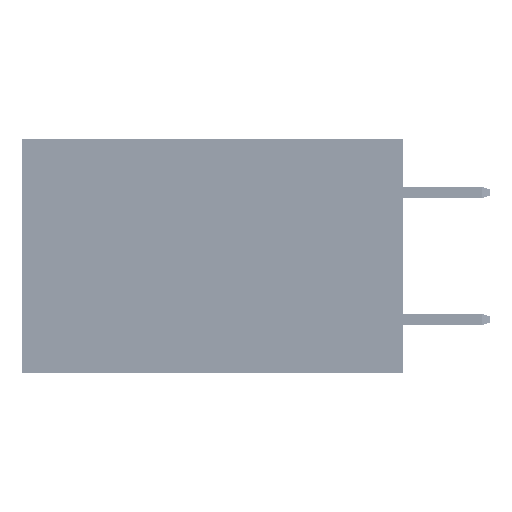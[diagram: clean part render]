
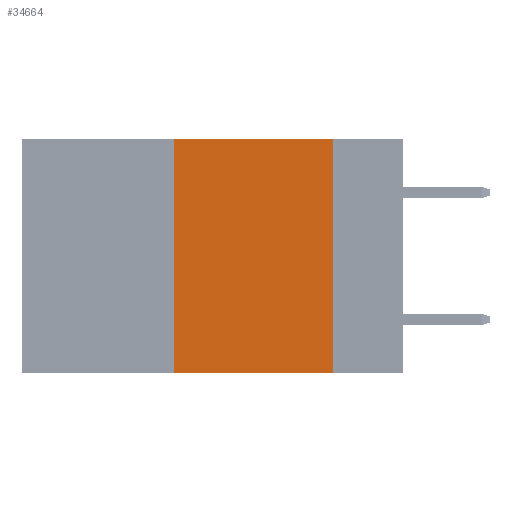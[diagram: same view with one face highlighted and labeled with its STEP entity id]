
A CAD part, left-side view. The second image highlights one B-rep face of the part: STEP entity #34664.
In plain terms, the highlighted planar face has unit normal (-1, 0, 0).
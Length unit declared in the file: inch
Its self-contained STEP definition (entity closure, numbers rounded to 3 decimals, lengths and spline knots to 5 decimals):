
#828 = CARTESIAN_POINT ( 'NONE',  ( 0., 0.11, -0.37 ) ) ;
#5156 = VERTEX_POINT ( 'NONE', #828 ) ;
#6216 = LINE ( 'NONE', #47493, #41495 ) ;
#6456 = DIRECTION ( 'NONE',  ( 0., 0., -1. ) ) ;
#7504 = DIRECTION ( 'NONE',  ( 0., -1., 0. ) ) ;
#7778 = DIRECTION ( 'NONE',  ( 0., 0., 1. ) ) ;
#10193 = DIRECTION ( 'NONE',  ( 0., 0., -1. ) ) ;
#11492 = LINE ( 'NONE', #42266, #32347 ) ;
#12004 = ORIENTED_EDGE ( 'NONE', *, *, #33417, .F. ) ;
#12226 = CARTESIAN_POINT ( 'NONE',  ( 0., 0.6, 0. ) ) ;
#13939 = EDGE_CURVE ( 'NONE', #21353, #24332, #30054, .T. ) ;
#15836 = DIRECTION ( 'NONE',  ( 0., -1., 0. ) ) ;
#15978 = FACE_OUTER_BOUND ( 'NONE', #25238, .T. ) ;
#20703 = EDGE_CURVE ( 'NONE', #21353, #5156, #11492, .T. ) ;
#21353 = VERTEX_POINT ( 'NONE', #43420 ) ;
#24332 = VERTEX_POINT ( 'NONE', #35027 ) ;
#25238 = EDGE_LOOP ( 'NONE', ( #12004, #46242, #26248, #47193 ) ) ;
#26248 = ORIENTED_EDGE ( 'NONE', *, *, #13939, .F. ) ;
#27470 = DIRECTION ( 'NONE',  ( 1., 0., 0. ) ) ;
#29247 = VERTEX_POINT ( 'NONE', #33492 ) ;
#30054 = LINE ( 'NONE', #41314, #41631 ) ;
#30618 = LINE ( 'NONE', #42126, #39050 ) ;
#31260 = PLANE ( 'NONE',  #42469 ) ;
#32347 = VECTOR ( 'NONE', #7504, 39.37008 ) ;
#33417 = EDGE_CURVE ( 'NONE', #29247, #5156, #6216, .T. ) ;
#33492 = CARTESIAN_POINT ( 'NONE',  ( 0., 0.11, 0. ) ) ;
#34664 = ADVANCED_FACE ( 'NONE', ( #15978 ), #31260, .F. ) ;
#35027 = CARTESIAN_POINT ( 'NONE',  ( 0., 0.36, 0. ) ) ;
#39050 = VECTOR ( 'NONE', #15836, 39.37008 ) ;
#41314 = CARTESIAN_POINT ( 'NONE',  ( 0., 0.36, 0. ) ) ;
#41495 = VECTOR ( 'NONE', #10193, 39.37008 ) ;
#41631 = VECTOR ( 'NONE', #7778, 39.37008 ) ;
#42126 = CARTESIAN_POINT ( 'NONE',  ( 0., 0.6, 0. ) ) ;
#42266 = CARTESIAN_POINT ( 'NONE',  ( 0., 0.6, -0.37 ) ) ;
#42469 = AXIS2_PLACEMENT_3D ( 'NONE', #12226, #27470, #6456 ) ;
#43420 = CARTESIAN_POINT ( 'NONE',  ( 0., 0.36, -0.37 ) ) ;
#46242 = ORIENTED_EDGE ( 'NONE', *, *, #46624, .F. ) ;
#46624 = EDGE_CURVE ( 'NONE', #24332, #29247, #30618, .T. ) ;
#47193 = ORIENTED_EDGE ( 'NONE', *, *, #20703, .T. ) ;
#47493 = CARTESIAN_POINT ( 'NONE',  ( 0., 0.11, 0. ) ) ;
